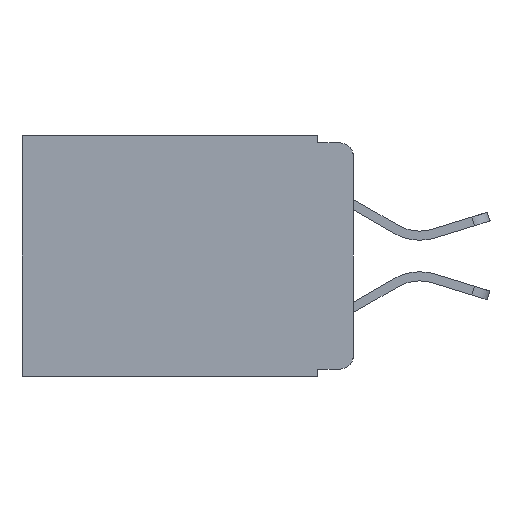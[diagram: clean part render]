
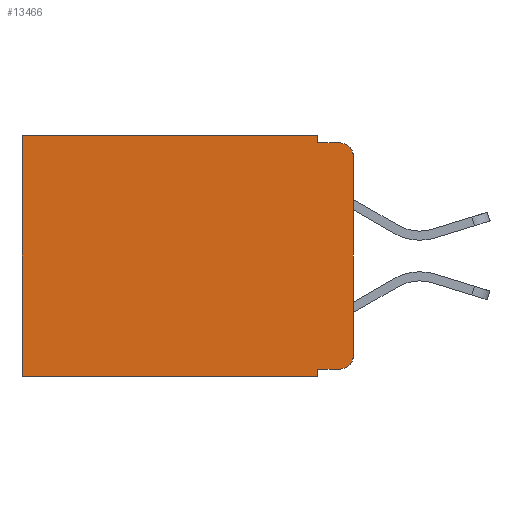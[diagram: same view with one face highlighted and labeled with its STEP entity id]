
A CAD part, left-side view. The second image highlights one B-rep face of the part: STEP entity #13466.
In plain terms, the highlighted planar face has unit normal (-1, 0, 0).
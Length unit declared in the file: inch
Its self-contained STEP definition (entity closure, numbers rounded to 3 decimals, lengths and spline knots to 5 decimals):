
#350 = ORIENTED_EDGE ( 'NONE', *, *, #11811, .T. ) ;
#364 = CARTESIAN_POINT ( 'NONE',  ( 0.298, 0.051, 0. ) ) ;
#845 = CARTESIAN_POINT ( 'NONE',  ( 0.298, 0., 0. ) ) ;
#904 = CIRCLE ( 'NONE', #20810, 0.02 ) ;
#1781 = EDGE_CURVE ( 'NONE', #13112, #18500, #8645, .T. ) ;
#2024 = EDGE_LOOP ( 'NONE', ( #23145, #6602, #10711, #12647, #6984, #14719, #14129, #15321, #350, #14248 ) ) ;
#2104 = CARTESIAN_POINT ( 'NONE',  ( 0.298, 0.051, 0. ) ) ;
#2189 = CARTESIAN_POINT ( 'NONE',  ( 0.298, 0.051, -0.343 ) ) ;
#3376 = EDGE_CURVE ( 'NONE', #3753, #23551, #22974, .T. ) ;
#3709 = CARTESIAN_POINT ( 'NONE',  ( 0.298, 0., -0.03 ) ) ;
#3753 = VERTEX_POINT ( 'NONE', #9458 ) ;
#4246 = DIRECTION ( 'NONE',  ( 1., 0., 0. ) ) ;
#4364 = PLANE ( 'NONE',  #8876 ) ;
#4989 = VERTEX_POINT ( 'NONE', #11610 ) ;
#5110 = CIRCLE ( 'NONE', #12919, 0.02 ) ;
#5122 = VECTOR ( 'NONE', #16009, 39.37008 ) ;
#6411 = LINE ( 'NONE', #19447, #16106 ) ;
#6602 = ORIENTED_EDGE ( 'NONE', *, *, #23930, .T. ) ;
#6631 = LINE ( 'NONE', #19672, #12391 ) ;
#6984 = ORIENTED_EDGE ( 'NONE', *, *, #23415, .T. ) ;
#7109 = VERTEX_POINT ( 'NONE', #16952 ) ;
#8131 = CARTESIAN_POINT ( 'NONE',  ( 0.298, 0., 0. ) ) ;
#8180 = LINE ( 'NONE', #845, #9670 ) ;
#8563 = VECTOR ( 'NONE', #11714, 39.37008 ) ;
#8586 = DIRECTION ( 'NONE',  ( 0., 1., 0. ) ) ;
#8645 = LINE ( 'NONE', #17920, #17163 ) ;
#8717 = VECTOR ( 'NONE', #11011, 39.37008 ) ;
#8876 = AXIS2_PLACEMENT_3D ( 'NONE', #8131, #4246, #13984 ) ;
#8912 = LINE ( 'NONE', #19890, #5122 ) ;
#9131 = CARTESIAN_POINT ( 'NONE',  ( 0.298, 0.02, -0.03 ) ) ;
#9183 = LINE ( 'NONE', #2104, #8717 ) ;
#9194 = EDGE_CURVE ( 'NONE', #12857, #18500, #6631, .T. ) ;
#9366 = DIRECTION ( 'NONE',  ( -1., 0., 0. ) ) ;
#9458 = CARTESIAN_POINT ( 'NONE',  ( 0.298, 0.051, 0. ) ) ;
#9648 = EDGE_CURVE ( 'NONE', #16819, #4989, #8180, .T. ) ;
#9670 = VECTOR ( 'NONE', #21516, 39.37008 ) ;
#10711 = ORIENTED_EDGE ( 'NONE', *, *, #22064, .F. ) ;
#10957 = DIRECTION ( 'NONE',  ( 0., 0., -1. ) ) ;
#11011 = DIRECTION ( 'NONE',  ( 0., 0., -1. ) ) ;
#11077 = DIRECTION ( 'NONE',  ( 0., 0., -1. ) ) ;
#11610 = CARTESIAN_POINT ( 'NONE',  ( 0.298, 0., -0.313 ) ) ;
#11714 = DIRECTION ( 'NONE',  ( 0., 0., -1. ) ) ;
#11811 = EDGE_CURVE ( 'NONE', #7109, #12318, #14581, .T. ) ;
#12001 = CARTESIAN_POINT ( 'NONE',  ( 0.298, 0.02, -0.01 ) ) ;
#12318 = VERTEX_POINT ( 'NONE', #18211 ) ;
#12391 = VECTOR ( 'NONE', #13706, 39.37008 ) ;
#12647 = ORIENTED_EDGE ( 'NONE', *, *, #3376, .F. ) ;
#12857 = VERTEX_POINT ( 'NONE', #2189 ) ;
#12919 = AXIS2_PLACEMENT_3D ( 'NONE', #16591, #20101, #16710 ) ;
#13112 = VERTEX_POINT ( 'NONE', #15971 ) ;
#13269 = VECTOR ( 'NONE', #16059, 39.37008 ) ;
#13466 = ADVANCED_FACE ( 'NONE', ( #17293 ), #4364, .F. ) ;
#13706 = DIRECTION ( 'NONE',  ( 0., 1., 0. ) ) ;
#13984 = DIRECTION ( 'NONE',  ( 0., 0., -1. ) ) ;
#14129 = ORIENTED_EDGE ( 'NONE', *, *, #9194, .F. ) ;
#14248 = ORIENTED_EDGE ( 'NONE', *, *, #21377, .T. ) ;
#14581 = LINE ( 'NONE', #18001, #13269 ) ;
#14719 = ORIENTED_EDGE ( 'NONE', *, *, #1781, .T. ) ;
#15321 = ORIENTED_EDGE ( 'NONE', *, *, #15508, .F. ) ;
#15508 = EDGE_CURVE ( 'NONE', #7109, #12857, #9183, .T. ) ;
#15971 = CARTESIAN_POINT ( 'NONE',  ( 0.298, 0.473, 0. ) ) ;
#16009 = DIRECTION ( 'NONE',  ( 0., -1., 0. ) ) ;
#16059 = DIRECTION ( 'NONE',  ( 0., -1., 0. ) ) ;
#16106 = VECTOR ( 'NONE', #8586, 39.37008 ) ;
#16591 = CARTESIAN_POINT ( 'NONE',  ( 0.298, 0.02, -0.313 ) ) ;
#16710 = DIRECTION ( 'NONE',  ( 0., 0., -1. ) ) ;
#16819 = VERTEX_POINT ( 'NONE', #3709 ) ;
#16952 = CARTESIAN_POINT ( 'NONE',  ( 0.298, 0.051, -0.333 ) ) ;
#17163 = VECTOR ( 'NONE', #10957, 39.37008 ) ;
#17293 = FACE_OUTER_BOUND ( 'NONE', #2024, .T. ) ;
#17920 = CARTESIAN_POINT ( 'NONE',  ( 0.298, 0.473, 0. ) ) ;
#18001 = CARTESIAN_POINT ( 'NONE',  ( 0.298, 0.051, -0.333 ) ) ;
#18211 = CARTESIAN_POINT ( 'NONE',  ( 0.298, 0.02, -0.333 ) ) ;
#18500 = VERTEX_POINT ( 'NONE', #21478 ) ;
#18945 = CARTESIAN_POINT ( 'NONE',  ( 0.298, 0.051, -0.01 ) ) ;
#19447 = CARTESIAN_POINT ( 'NONE',  ( 0.298, 0., 0. ) ) ;
#19672 = CARTESIAN_POINT ( 'NONE',  ( 0.298, 0., -0.343 ) ) ;
#19890 = CARTESIAN_POINT ( 'NONE',  ( 0.298, 0.051, -0.01 ) ) ;
#20101 = DIRECTION ( 'NONE',  ( -1., 0., 0. ) ) ;
#20810 = AXIS2_PLACEMENT_3D ( 'NONE', #9131, #9366, #11077 ) ;
#21377 = EDGE_CURVE ( 'NONE', #12318, #4989, #5110, .T. ) ;
#21478 = CARTESIAN_POINT ( 'NONE',  ( 0.298, 0.473, -0.343 ) ) ;
#21516 = DIRECTION ( 'NONE',  ( 0., 0., -1. ) ) ;
#22064 = EDGE_CURVE ( 'NONE', #23551, #23362, #8912, .T. ) ;
#22974 = LINE ( 'NONE', #364, #8563 ) ;
#23145 = ORIENTED_EDGE ( 'NONE', *, *, #9648, .F. ) ;
#23362 = VERTEX_POINT ( 'NONE', #12001 ) ;
#23415 = EDGE_CURVE ( 'NONE', #3753, #13112, #6411, .T. ) ;
#23551 = VERTEX_POINT ( 'NONE', #18945 ) ;
#23930 = EDGE_CURVE ( 'NONE', #16819, #23362, #904, .T. ) ;
